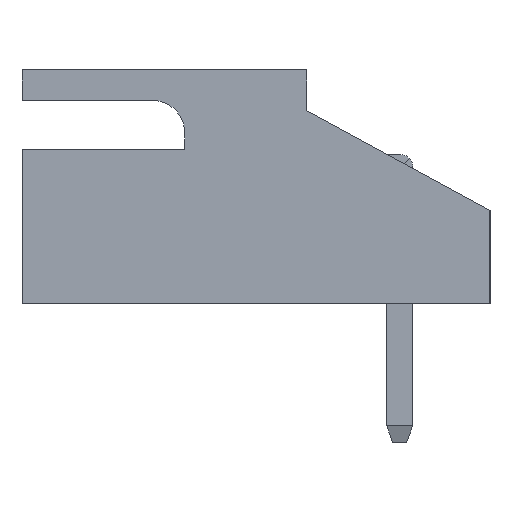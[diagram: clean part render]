
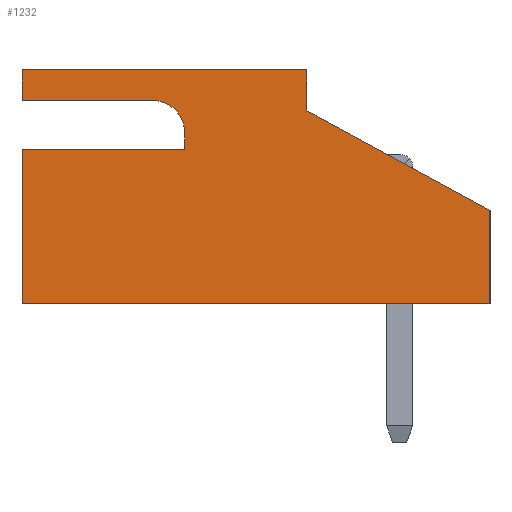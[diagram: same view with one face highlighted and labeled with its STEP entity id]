
A CAD part, left-side view. The second image highlights one B-rep face of the part: STEP entity #1232.
In plain terms, the highlighted planar face has unit normal (-1, 0, 0).
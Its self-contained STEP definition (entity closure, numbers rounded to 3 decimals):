
#27 = CARTESIAN_POINT ( 'NONE',  ( -12.5, 0., 1.875 ) ) ;
#83 = CARTESIAN_POINT ( 'NONE',  ( -12.5, 3., 0.925 ) ) ;
#87 = VECTOR ( 'NONE', #4035, 1000. ) ;
#150 = CARTESIAN_POINT ( 'NONE',  ( -12.5, 7., -2.875 ) ) ;
#239 = CARTESIAN_POINT ( 'NONE',  ( -12.5, 7., 2.875 ) ) ;
#297 = CARTESIAN_POINT ( 'NONE',  ( -12.5, 0., -2.875 ) ) ;
#327 = VERTEX_POINT ( 'NONE', #3299 ) ;
#381 = ORIENTED_EDGE ( 'NONE', *, *, #2720, .T. ) ;
#401 = CARTESIAN_POINT ( 'NONE',  ( -12.5, 7., 0.925 ) ) ;
#430 = EDGE_CURVE ( 'NONE', #2520, #1014, #5115, .T. ) ;
#489 = VERTEX_POINT ( 'NONE', #401 ) ;
#546 = VECTOR ( 'NONE', #5274, 1000. ) ;
#577 = LINE ( 'NONE', #2866, #4048 ) ;
#632 = DIRECTION ( 'NONE',  ( 0., 0., 1. ) ) ;
#674 = ORIENTED_EDGE ( 'NONE', *, *, #3422, .T. ) ;
#694 = EDGE_LOOP ( 'NONE', ( #2804, #4795, #1691, #381, #674, #1744, #857, #2981, #4275, #2144, #2785 ) ) ;
#717 = VECTOR ( 'NONE', #2017, 1000. ) ;
#835 = VECTOR ( 'NONE', #2807, 1000. ) ;
#857 = ORIENTED_EDGE ( 'NONE', *, *, #1353, .T. ) ;
#894 = VECTOR ( 'NONE', #2319, 1000. ) ;
#1014 = VERTEX_POINT ( 'NONE', #3607 ) ;
#1060 = DIRECTION ( 'NONE',  ( 0., 1., 0. ) ) ;
#1061 = CARTESIAN_POINT ( 'NONE',  ( -12.5, 3., 1.325 ) ) ;
#1084 = AXIS2_PLACEMENT_3D ( 'NONE', #1107, #5568, #4218 ) ;
#1107 = CARTESIAN_POINT ( 'NONE',  ( -12.5, 7., -2.875 ) ) ;
#1232 = ADVANCED_FACE ( 'NONE', ( #2455 ), #5596, .F. ) ;
#1353 = EDGE_CURVE ( 'NONE', #4319, #4495, #5677, .T. ) ;
#1369 = CIRCLE ( 'NONE', #4855, 0.8 ) ;
#1578 = VECTOR ( 'NONE', #2688, 1000. ) ;
#1691 = ORIENTED_EDGE ( 'NONE', *, *, #3604, .T. ) ;
#1744 = ORIENTED_EDGE ( 'NONE', *, *, #4347, .F. ) ;
#1953 = LINE ( 'NONE', #4995, #835 ) ;
#2017 = DIRECTION ( 'NONE',  ( 0., 0., -1. ) ) ;
#2090 = VECTOR ( 'NONE', #1060, 1000. ) ;
#2144 = ORIENTED_EDGE ( 'NONE', *, *, #5276, .T. ) ;
#2319 = DIRECTION ( 'NONE',  ( 0., -1., 0. ) ) ;
#2455 = FACE_OUTER_BOUND ( 'NONE', #694, .T. ) ;
#2491 = VERTEX_POINT ( 'NONE', #27 ) ;
#2501 = CARTESIAN_POINT ( 'NONE',  ( -12.5, 7., 2.875 ) ) ;
#2520 = VERTEX_POINT ( 'NONE', #239 ) ;
#2630 = VERTEX_POINT ( 'NONE', #1061 ) ;
#2688 = DIRECTION ( 'NONE',  ( 0., -0.878, -0.478 ) ) ;
#2720 = EDGE_CURVE ( 'NONE', #2630, #4615, #5090, .T. ) ;
#2785 = ORIENTED_EDGE ( 'NONE', *, *, #430, .F. ) ;
#2804 = ORIENTED_EDGE ( 'NONE', *, *, #3777, .F. ) ;
#2807 = DIRECTION ( 'NONE',  ( 0., 0., -1. ) ) ;
#2866 = CARTESIAN_POINT ( 'NONE',  ( -12.5, 7., -2.875 ) ) ;
#2968 = DIRECTION ( 'NONE',  ( 1., 0., 0. ) ) ;
#2981 = ORIENTED_EDGE ( 'NONE', *, *, #4317, .F. ) ;
#3044 = LINE ( 'NONE', #297, #5436 ) ;
#3057 = CARTESIAN_POINT ( 'NONE',  ( -12.5, 0., 1.875 ) ) ;
#3136 = LINE ( 'NONE', #4460, #87 ) ;
#3142 = EDGE_CURVE ( 'NONE', #327, #5445, #4872, .T. ) ;
#3299 = CARTESIAN_POINT ( 'NONE',  ( -12.5, 7., 2.125 ) ) ;
#3414 = CARTESIAN_POINT ( 'NONE',  ( -12.5, -4.5, -2.875 ) ) ;
#3422 = EDGE_CURVE ( 'NONE', #4615, #489, #4056, .T. ) ;
#3424 = CARTESIAN_POINT ( 'NONE',  ( -12.5, 3.8, 1.325 ) ) ;
#3604 = EDGE_CURVE ( 'NONE', #5445, #2630, #1369, .T. ) ;
#3607 = CARTESIAN_POINT ( 'NONE',  ( -12.5, 0., 2.875 ) ) ;
#3777 = EDGE_CURVE ( 'NONE', #327, #2520, #3136, .T. ) ;
#3941 = CARTESIAN_POINT ( 'NONE',  ( -12.5, 7., 0.925 ) ) ;
#4035 = DIRECTION ( 'NONE',  ( 0., 0., 1. ) ) ;
#4048 = VECTOR ( 'NONE', #632, 1000. ) ;
#4056 = LINE ( 'NONE', #3941, #2090 ) ;
#4122 = VECTOR ( 'NONE', #5609, 1000. ) ;
#4218 = DIRECTION ( 'NONE',  ( 0., 0., -1. ) ) ;
#4275 = ORIENTED_EDGE ( 'NONE', *, *, #5023, .F. ) ;
#4317 = EDGE_CURVE ( 'NONE', #4701, #4495, #1953, .T. ) ;
#4319 = VERTEX_POINT ( 'NONE', #150 ) ;
#4332 = CARTESIAN_POINT ( 'NONE',  ( -12.5, 7., -2.875 ) ) ;
#4347 = EDGE_CURVE ( 'NONE', #4319, #489, #577, .T. ) ;
#4371 = CARTESIAN_POINT ( 'NONE',  ( -12.5, -4.5, -0.575 ) ) ;
#4460 = CARTESIAN_POINT ( 'NONE',  ( -12.5, 7., -2.875 ) ) ;
#4495 = VERTEX_POINT ( 'NONE', #3414 ) ;
#4615 = VERTEX_POINT ( 'NONE', #83 ) ;
#4701 = VERTEX_POINT ( 'NONE', #4371 ) ;
#4717 = DIRECTION ( 'NONE',  ( 0., 0., 1. ) ) ;
#4772 = CARTESIAN_POINT ( 'NONE',  ( -12.5, 3.8, 2.125 ) ) ;
#4795 = ORIENTED_EDGE ( 'NONE', *, *, #3142, .T. ) ;
#4855 = AXIS2_PLACEMENT_3D ( 'NONE', #3424, #2968, #5182 ) ;
#4872 = LINE ( 'NONE', #4983, #894 ) ;
#4983 = CARTESIAN_POINT ( 'NONE',  ( -12.5, 7., 2.125 ) ) ;
#4995 = CARTESIAN_POINT ( 'NONE',  ( -12.5, -4.5, -0.575 ) ) ;
#5023 = EDGE_CURVE ( 'NONE', #2491, #4701, #5224, .T. ) ;
#5090 = LINE ( 'NONE', #5528, #717 ) ;
#5115 = LINE ( 'NONE', #2501, #4122 ) ;
#5182 = DIRECTION ( 'NONE',  ( 0., 0., -1. ) ) ;
#5224 = LINE ( 'NONE', #3057, #1578 ) ;
#5274 = DIRECTION ( 'NONE',  ( 0., -1., 0. ) ) ;
#5276 = EDGE_CURVE ( 'NONE', #2491, #1014, #3044, .T. ) ;
#5436 = VECTOR ( 'NONE', #4717, 1000. ) ;
#5445 = VERTEX_POINT ( 'NONE', #4772 ) ;
#5528 = CARTESIAN_POINT ( 'NONE',  ( -12.5, 3., 1.325 ) ) ;
#5568 = DIRECTION ( 'NONE',  ( 1., 0., 0. ) ) ;
#5596 = PLANE ( 'NONE',  #1084 ) ;
#5609 = DIRECTION ( 'NONE',  ( 0., -1., 0. ) ) ;
#5677 = LINE ( 'NONE', #4332, #546 ) ;
